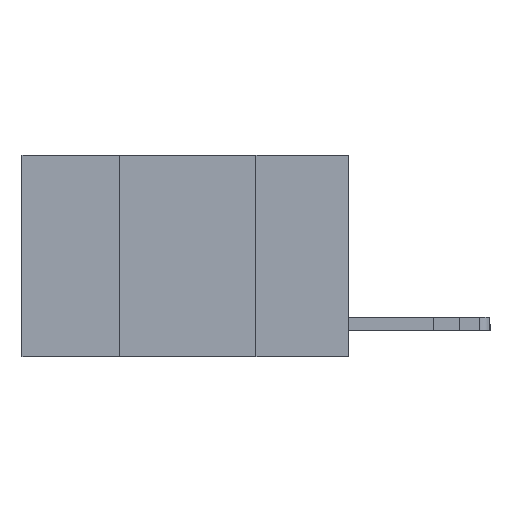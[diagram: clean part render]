
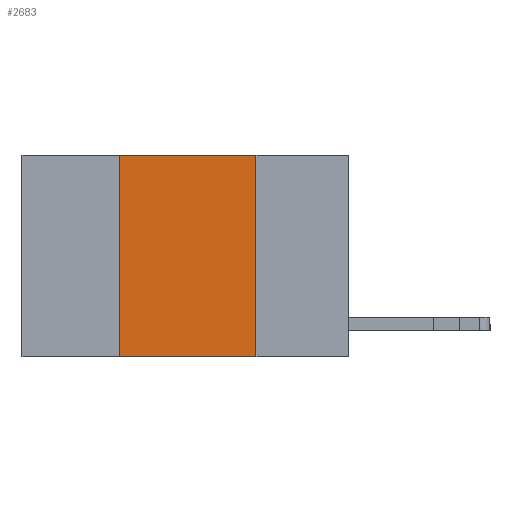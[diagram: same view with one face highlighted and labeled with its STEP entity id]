
A CAD part, left-side view. The second image highlights one B-rep face of the part: STEP entity #2683.
In plain terms, the highlighted planar face has unit normal (-1, 0, 0).
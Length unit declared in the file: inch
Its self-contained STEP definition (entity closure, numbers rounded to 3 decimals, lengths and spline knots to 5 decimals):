
#1311 = LINE ( 'NONE', #19666, #17087 ) ;
#1507 = LINE ( 'NONE', #4713, #19130 ) ;
#2597 = DIRECTION ( 'NONE',  ( 0., 0., 1. ) ) ;
#2683 = ADVANCED_FACE ( 'NONE', ( #7658 ), #10612, .F. ) ;
#3229 = CARTESIAN_POINT ( 'NONE',  ( 0., 0.42, -0.37 ) ) ;
#3621 = ORIENTED_EDGE ( 'NONE', *, *, #4563, .F. ) ;
#4307 = LINE ( 'NONE', #13745, #19403 ) ;
#4423 = CARTESIAN_POINT ( 'NONE',  ( 0., 0.42, 0. ) ) ;
#4563 = EDGE_CURVE ( 'NONE', #15715, #6233, #1311, .T. ) ;
#4713 = CARTESIAN_POINT ( 'NONE',  ( 0., 0.17, 0. ) ) ;
#5391 = ORIENTED_EDGE ( 'NONE', *, *, #21017, .F. ) ;
#6233 = VERTEX_POINT ( 'NONE', #14455 ) ;
#6612 = VERTEX_POINT ( 'NONE', #20102 ) ;
#7658 = FACE_OUTER_BOUND ( 'NONE', #18005, .T. ) ;
#7697 = DIRECTION ( 'NONE',  ( 0., -1., 0. ) ) ;
#10612 = PLANE ( 'NONE',  #13342 ) ;
#10629 = VERTEX_POINT ( 'NONE', #3229 ) ;
#11021 = ORIENTED_EDGE ( 'NONE', *, *, #11896, .F. ) ;
#11896 = EDGE_CURVE ( 'NONE', #10629, #15715, #4307, .T. ) ;
#12517 = DIRECTION ( 'NONE',  ( 1., 0., 0. ) ) ;
#13126 = ORIENTED_EDGE ( 'NONE', *, *, #16567, .T. ) ;
#13342 = AXIS2_PLACEMENT_3D ( 'NONE', #13807, #12517, #15506 ) ;
#13451 = DIRECTION ( 'NONE',  ( 0., -1., 0. ) ) ;
#13528 = VECTOR ( 'NONE', #13451, 39.37008 ) ;
#13745 = CARTESIAN_POINT ( 'NONE',  ( 0., 0.42, 0. ) ) ;
#13776 = CARTESIAN_POINT ( 'NONE',  ( 0., 0.6, -0.37 ) ) ;
#13807 = CARTESIAN_POINT ( 'NONE',  ( 0., 0.6, 0. ) ) ;
#14455 = CARTESIAN_POINT ( 'NONE',  ( 0., 0.17, 0. ) ) ;
#15506 = DIRECTION ( 'NONE',  ( 0., 0., -1. ) ) ;
#15715 = VERTEX_POINT ( 'NONE', #4423 ) ;
#16567 = EDGE_CURVE ( 'NONE', #10629, #6612, #16754, .T. ) ;
#16754 = LINE ( 'NONE', #13776, #13528 ) ;
#17087 = VECTOR ( 'NONE', #7697, 39.37008 ) ;
#18005 = EDGE_LOOP ( 'NONE', ( #5391, #3621, #11021, #13126 ) ) ;
#19130 = VECTOR ( 'NONE', #19473, 39.37008 ) ;
#19403 = VECTOR ( 'NONE', #2597, 39.37008 ) ;
#19473 = DIRECTION ( 'NONE',  ( 0., 0., -1. ) ) ;
#19666 = CARTESIAN_POINT ( 'NONE',  ( 0., 0.6, 0. ) ) ;
#20102 = CARTESIAN_POINT ( 'NONE',  ( 0., 0.17, -0.37 ) ) ;
#21017 = EDGE_CURVE ( 'NONE', #6233, #6612, #1507, .T. ) ;
